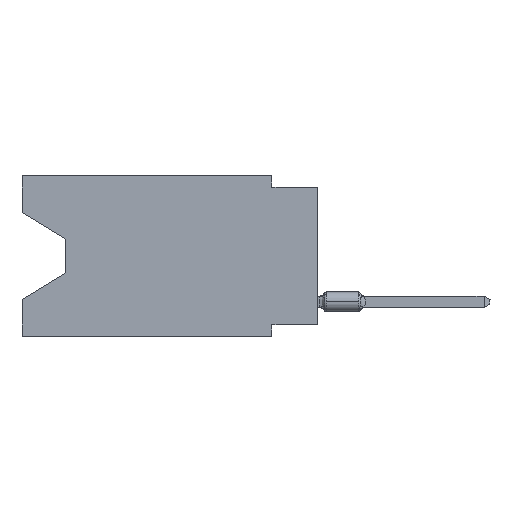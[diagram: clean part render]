
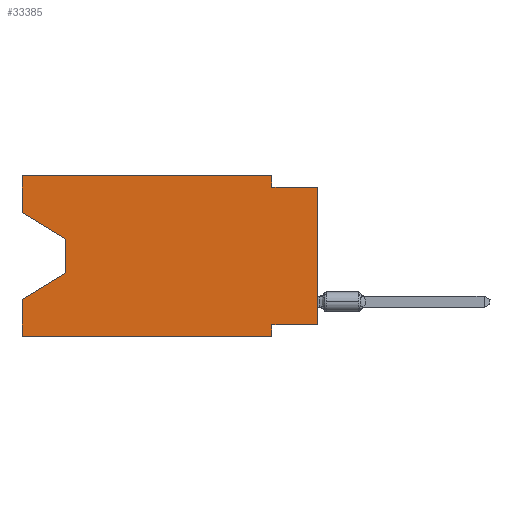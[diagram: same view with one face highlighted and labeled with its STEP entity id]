
A CAD part, left-side view. The second image highlights one B-rep face of the part: STEP entity #33385.
In plain terms, the highlighted planar face has unit normal (-1, 0, 0).
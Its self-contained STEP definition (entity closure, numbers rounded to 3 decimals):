
#1677 = CARTESIAN_POINT ( 'NONE',  ( 0., 0., -0.635 ) ) ;
#3252 = VERTEX_POINT ( 'NONE', #8071 ) ;
#3862 = CARTESIAN_POINT ( 'NONE',  ( 0., 16.383, -2.038 ) ) ;
#4261 = CARTESIAN_POINT ( 'NONE',  ( 0., 13.97, -5.385 ) ) ;
#4651 = DIRECTION ( 'NONE',  ( 0., 0.855, -0.519 ) ) ;
#5023 = LINE ( 'NONE', #4261, #40983 ) ;
#5379 = VECTOR ( 'NONE', #32513, 1000. ) ;
#5714 = CARTESIAN_POINT ( 'NONE',  ( 0., 13.97, -3.505 ) ) ;
#6352 = EDGE_CURVE ( 'NONE', #33158, #71298, #33843, .T. ) ;
#6362 = DIRECTION ( 'NONE',  ( 0., 0., -1. ) ) ;
#7294 = LINE ( 'NONE', #47419, #63382 ) ;
#8071 = CARTESIAN_POINT ( 'NONE',  ( 0., 0., -0.635 ) ) ;
#9540 = ORIENTED_EDGE ( 'NONE', *, *, #70969, .F. ) ;
#11004 = VECTOR ( 'NONE', #33472, 1000. ) ;
#13574 = DIRECTION ( 'NONE',  ( 0., 1., 0. ) ) ;
#13679 = DIRECTION ( 'NONE',  ( 0., -1., 0. ) ) ;
#13949 = VECTOR ( 'NONE', #73959, 1000. ) ;
#15419 = ORIENTED_EDGE ( 'NONE', *, *, #70680, .T. ) ;
#15928 = ORIENTED_EDGE ( 'NONE', *, *, #76071, .T. ) ;
#17256 = ORIENTED_EDGE ( 'NONE', *, *, #22816, .F. ) ;
#17927 = VECTOR ( 'NONE', #36347, 1000. ) ;
#18706 = VERTEX_POINT ( 'NONE', #73491 ) ;
#19094 = CARTESIAN_POINT ( 'NONE',  ( 0., 16.383, 0. ) ) ;
#19590 = ORIENTED_EDGE ( 'NONE', *, *, #62870, .F. ) ;
#20292 = CARTESIAN_POINT ( 'NONE',  ( 0., 2.54, 0. ) ) ;
#21683 = ORIENTED_EDGE ( 'NONE', *, *, #21962, .T. ) ;
#21934 = DIRECTION ( 'NONE',  ( 0., 0., -1. ) ) ;
#21962 = EDGE_CURVE ( 'NONE', #65316, #3252, #42755, .T. ) ;
#22811 = EDGE_LOOP ( 'NONE', ( #60184, #15419, #53698, #43444, #15928, #9540, #29558, #21683, #17256, #50103, #19590, #40792 ) ) ;
#22816 = EDGE_CURVE ( 'NONE', #41445, #3252, #61966, .T. ) ;
#23146 = EDGE_CURVE ( 'NONE', #33158, #37950, #74296, .T. ) ;
#23410 = CARTESIAN_POINT ( 'NONE',  ( 0., 0., 0. ) ) ;
#24503 = CARTESIAN_POINT ( 'NONE',  ( 0., 2.54, -8.89 ) ) ;
#25571 = EDGE_CURVE ( 'NONE', #50387, #18706, #5023, .T. ) ;
#27377 = CARTESIAN_POINT ( 'NONE',  ( 0., 16.383, -8.89 ) ) ;
#28551 = CARTESIAN_POINT ( 'NONE',  ( 0., 16.383, 0. ) ) ;
#29054 = DIRECTION ( 'NONE',  ( 0., 0., -1. ) ) ;
#29558 = ORIENTED_EDGE ( 'NONE', *, *, #44616, .F. ) ;
#30854 = CARTESIAN_POINT ( 'NONE',  ( 0., 2.54, -0.635 ) ) ;
#32513 = DIRECTION ( 'NONE',  ( 0., 0., -1. ) ) ;
#33158 = VERTEX_POINT ( 'NONE', #37930 ) ;
#33385 = ADVANCED_FACE ( 'NONE', ( #64383 ), #58165, .F. ) ;
#33472 = DIRECTION ( 'NONE',  ( 0., -1., 0. ) ) ;
#33843 = LINE ( 'NONE', #57602, #13949 ) ;
#34006 = VECTOR ( 'NONE', #21934, 1000. ) ;
#35668 = VERTEX_POINT ( 'NONE', #27377 ) ;
#36099 = VERTEX_POINT ( 'NONE', #20292 ) ;
#36347 = DIRECTION ( 'NONE',  ( 0., 0., 1. ) ) ;
#37930 = CARTESIAN_POINT ( 'NONE',  ( 0., 16.383, -2.038 ) ) ;
#37950 = VERTEX_POINT ( 'NONE', #41574 ) ;
#40682 = VECTOR ( 'NONE', #51882, 1000. ) ;
#40792 = ORIENTED_EDGE ( 'NONE', *, *, #6352, .F. ) ;
#40968 = LINE ( 'NONE', #45686, #34006 ) ;
#40983 = VECTOR ( 'NONE', #4651, 1000. ) ;
#41445 = VERTEX_POINT ( 'NONE', #30854 ) ;
#41574 = CARTESIAN_POINT ( 'NONE',  ( 0., 13.97, -3.505 ) ) ;
#42374 = VERTEX_POINT ( 'NONE', #58592 ) ;
#42755 = LINE ( 'NONE', #23410, #40682 ) ;
#43444 = ORIENTED_EDGE ( 'NONE', *, *, #53980, .F. ) ;
#44616 = EDGE_CURVE ( 'NONE', #65316, #42374, #56022, .T. ) ;
#45686 = CARTESIAN_POINT ( 'NONE',  ( 0., 2.54, 0. ) ) ;
#46210 = LINE ( 'NONE', #5714, #68666 ) ;
#46787 = VECTOR ( 'NONE', #13679, 1000. ) ;
#47280 = LINE ( 'NONE', #71016, #17927 ) ;
#47419 = CARTESIAN_POINT ( 'NONE',  ( 0., 16.383, 0. ) ) ;
#49435 = CARTESIAN_POINT ( 'NONE',  ( 0., 0., -8.255 ) ) ;
#50103 = ORIENTED_EDGE ( 'NONE', *, *, #52759, .F. ) ;
#50387 = VERTEX_POINT ( 'NONE', #65843 ) ;
#50525 = VECTOR ( 'NONE', #13574, 1000. ) ;
#51016 = CARTESIAN_POINT ( 'NONE',  ( 0., 16.383, -8.89 ) ) ;
#51787 = LINE ( 'NONE', #51016, #11004 ) ;
#51882 = DIRECTION ( 'NONE',  ( 0., 0., 1. ) ) ;
#52759 = EDGE_CURVE ( 'NONE', #36099, #41445, #40968, .T. ) ;
#53404 = VERTEX_POINT ( 'NONE', #24503 ) ;
#53698 = ORIENTED_EDGE ( 'NONE', *, *, #25571, .T. ) ;
#53980 = EDGE_CURVE ( 'NONE', #35668, #18706, #47280, .T. ) ;
#55565 = VECTOR ( 'NONE', #63023, 1000. ) ;
#56022 = LINE ( 'NONE', #49435, #50525 ) ;
#57602 = CARTESIAN_POINT ( 'NONE',  ( 0., 16.383, 0. ) ) ;
#58165 = PLANE ( 'NONE',  #66044 ) ;
#58592 = CARTESIAN_POINT ( 'NONE',  ( 0., 2.54, -8.255 ) ) ;
#59691 = DIRECTION ( 'NONE',  ( 1., 0., 0. ) ) ;
#60184 = ORIENTED_EDGE ( 'NONE', *, *, #23146, .T. ) ;
#61720 = CARTESIAN_POINT ( 'NONE',  ( 0., 2.54, -8.89 ) ) ;
#61966 = LINE ( 'NONE', #1677, #46787 ) ;
#62870 = EDGE_CURVE ( 'NONE', #71298, #36099, #7294, .T. ) ;
#63023 = DIRECTION ( 'NONE',  ( 0., -0.855, -0.519 ) ) ;
#63382 = VECTOR ( 'NONE', #71150, 1000. ) ;
#64383 = FACE_OUTER_BOUND ( 'NONE', #22811, .T. ) ;
#65316 = VERTEX_POINT ( 'NONE', #72030 ) ;
#65843 = CARTESIAN_POINT ( 'NONE',  ( 0., 13.97, -5.385 ) ) ;
#66044 = AXIS2_PLACEMENT_3D ( 'NONE', #28551, #59691, #6362 ) ;
#68666 = VECTOR ( 'NONE', #29054, 1000. ) ;
#70680 = EDGE_CURVE ( 'NONE', #37950, #50387, #46210, .T. ) ;
#70969 = EDGE_CURVE ( 'NONE', #42374, #53404, #74924, .T. ) ;
#71016 = CARTESIAN_POINT ( 'NONE',  ( 0., 16.383, 0. ) ) ;
#71150 = DIRECTION ( 'NONE',  ( 0., -1., 0. ) ) ;
#71298 = VERTEX_POINT ( 'NONE', #19094 ) ;
#72030 = CARTESIAN_POINT ( 'NONE',  ( 0., 0., -8.255 ) ) ;
#73491 = CARTESIAN_POINT ( 'NONE',  ( 0., 16.383, -6.852 ) ) ;
#73959 = DIRECTION ( 'NONE',  ( 0., 0., 1. ) ) ;
#74296 = LINE ( 'NONE', #3862, #55565 ) ;
#74924 = LINE ( 'NONE', #61720, #5379 ) ;
#76071 = EDGE_CURVE ( 'NONE', #35668, #53404, #51787, .T. ) ;
